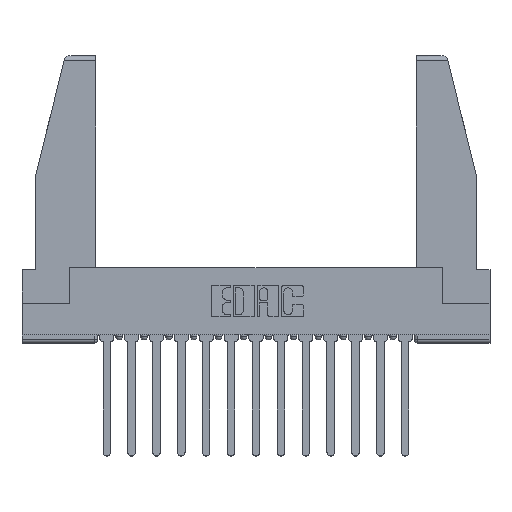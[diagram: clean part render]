
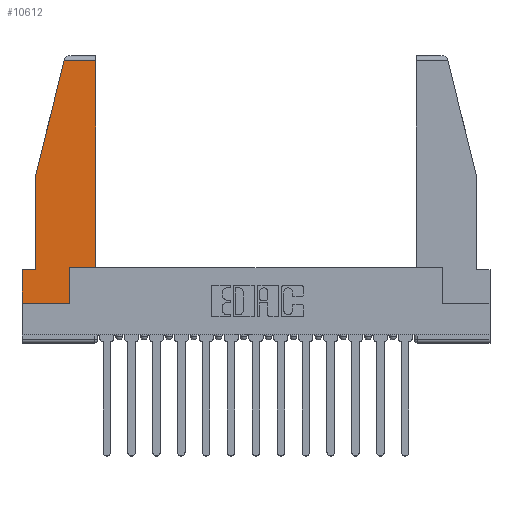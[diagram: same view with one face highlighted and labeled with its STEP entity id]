
A CAD part, top view. The second image highlights one B-rep face of the part: STEP entity #10612.
In plain terms, the highlighted planar face has unit normal (0, 0, 1).
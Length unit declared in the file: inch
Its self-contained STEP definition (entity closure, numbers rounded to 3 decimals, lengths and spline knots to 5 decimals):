
#54 = CARTESIAN_POINT ( 'NONE',  ( 0.086, 0.8, 0. ) ) ;
#259 = VECTOR ( 'NONE', #15701, 39.37008 ) ;
#649 = VECTOR ( 'NONE', #9842, 39.37008 ) ;
#1155 = EDGE_CURVE ( 'NONE', #9492, #9834, #7356, .T. ) ;
#1210 = CARTESIAN_POINT ( 'NONE',  ( 0., 0.21, 0. ) ) ;
#1335 = CARTESIAN_POINT ( 'NONE',  ( 0.086, 0.8, 0. ) ) ;
#1505 = ORIENTED_EDGE ( 'NONE', *, *, #7313, .T. ) ;
#1753 = DIRECTION ( 'NONE',  ( 0., 0., 1. ) ) ;
#2202 = CARTESIAN_POINT ( 'NONE',  ( 0., 0., 0. ) ) ;
#2274 = ORIENTED_EDGE ( 'NONE', *, *, #9126, .T. ) ;
#2557 = CARTESIAN_POINT ( 'NONE',  ( 0.297, 0., 0. ) ) ;
#2591 = VERTEX_POINT ( 'NONE', #7736 ) ;
#2814 = VERTEX_POINT ( 'NONE', #14049 ) ;
#3544 = VECTOR ( 'NONE', #5554, 39.37008 ) ;
#4175 = CARTESIAN_POINT ( 'NONE',  ( 0., 0.21, 0. ) ) ;
#4915 = LINE ( 'NONE', #11040, #16623 ) ;
#5093 = LINE ( 'NONE', #54, #8289 ) ;
#5324 = ORIENTED_EDGE ( 'NONE', *, *, #15727, .T. ) ;
#5519 = CARTESIAN_POINT ( 'NONE',  ( 0.461, 0.223, 0. ) ) ;
#5554 = DIRECTION ( 'NONE',  ( 0., -1., 0. ) ) ;
#5571 = CARTESIAN_POINT ( 'NONE',  ( 0., 1.52, 0. ) ) ;
#5779 = DIRECTION ( 'NONE',  ( 1., 0., 0. ) ) ;
#6099 = FACE_OUTER_BOUND ( 'NONE', #8479, .T. ) ;
#6162 = CARTESIAN_POINT ( 'NONE',  ( 0.086, 0.21, 0. ) ) ;
#6702 = DIRECTION ( 'NONE',  ( -1., 0., 0. ) ) ;
#7313 = EDGE_CURVE ( 'NONE', #2814, #13799, #17312, .T. ) ;
#7356 = LINE ( 'NONE', #4175, #3544 ) ;
#7708 = VERTEX_POINT ( 'NONE', #10818 ) ;
#7736 = CARTESIAN_POINT ( 'NONE',  ( 0.297, 0., 0. ) ) ;
#7889 = ORIENTED_EDGE ( 'NONE', *, *, #16744, .T. ) ;
#7936 = DIRECTION ( 'NONE',  ( 0., 1., 0. ) ) ;
#8087 = VECTOR ( 'NONE', #6702, 39.37008 ) ;
#8289 = VECTOR ( 'NONE', #10872, 39.37008 ) ;
#8439 = CARTESIAN_POINT ( 'NONE',  ( 0., 0.21, 0. ) ) ;
#8461 = LINE ( 'NONE', #15253, #649 ) ;
#8479 = EDGE_LOOP ( 'NONE', ( #2274, #5324, #10916, #12955, #14095, #17023, #15473, #7889, #1505 ) ) ;
#8797 = VECTOR ( 'NONE', #14078, 39.37008 ) ;
#9126 = EDGE_CURVE ( 'NONE', #13799, #16346, #9981, .T. ) ;
#9385 = EDGE_CURVE ( 'NONE', #14887, #15211, #5093, .T. ) ;
#9492 = VERTEX_POINT ( 'NONE', #8439 ) ;
#9834 = VERTEX_POINT ( 'NONE', #2202 ) ;
#9842 = DIRECTION ( 'NONE',  ( -0.239, -0.971, 0. ) ) ;
#9981 = LINE ( 'NONE', #11526, #259 ) ;
#10175 = EDGE_CURVE ( 'NONE', #7708, #14887, #8461, .T. ) ;
#10305 = LINE ( 'NONE', #2557, #11815 ) ;
#10612 = ADVANCED_FACE ( 'NONE', ( #6099 ), #16486, .T. ) ;
#10818 = CARTESIAN_POINT ( 'NONE',  ( 0.2636, 1.52, 0. ) ) ;
#10872 = DIRECTION ( 'NONE',  ( 0., -1., 0. ) ) ;
#10916 = ORIENTED_EDGE ( 'NONE', *, *, #10175, .T. ) ;
#11040 = CARTESIAN_POINT ( 'NONE',  ( 0., 0., 0. ) ) ;
#11102 = DIRECTION ( 'NONE',  ( 1., 0., 0. ) ) ;
#11526 = CARTESIAN_POINT ( 'NONE',  ( 0.461, 0.223, 0. ) ) ;
#11815 = VECTOR ( 'NONE', #7936, 39.37008 ) ;
#12280 = LINE ( 'NONE', #5571, #16309 ) ;
#12955 = ORIENTED_EDGE ( 'NONE', *, *, #9385, .T. ) ;
#13193 = EDGE_CURVE ( 'NONE', #9834, #2591, #4915, .T. ) ;
#13586 = EDGE_CURVE ( 'NONE', #15211, #9492, #13845, .T. ) ;
#13799 = VERTEX_POINT ( 'NONE', #5519 ) ;
#13845 = LINE ( 'NONE', #1210, #8087 ) ;
#14049 = CARTESIAN_POINT ( 'NONE',  ( 0.297, 0.223, 0. ) ) ;
#14078 = DIRECTION ( 'NONE',  ( 1., 0., 0. ) ) ;
#14095 = ORIENTED_EDGE ( 'NONE', *, *, #13586, .T. ) ;
#14887 = VERTEX_POINT ( 'NONE', #1335 ) ;
#15075 = DIRECTION ( 'NONE',  ( -1., 0., 0. ) ) ;
#15114 = AXIS2_PLACEMENT_3D ( 'NONE', #15168, #1753, #5779 ) ;
#15168 = CARTESIAN_POINT ( 'NONE',  ( 0., 0., 0. ) ) ;
#15211 = VERTEX_POINT ( 'NONE', #6162 ) ;
#15253 = CARTESIAN_POINT ( 'NONE',  ( 0.271, 1.55, 0. ) ) ;
#15473 = ORIENTED_EDGE ( 'NONE', *, *, #13193, .T. ) ;
#15668 = CARTESIAN_POINT ( 'NONE',  ( 0.297, 0.223, 0. ) ) ;
#15701 = DIRECTION ( 'NONE',  ( 0., 1., 0. ) ) ;
#15727 = EDGE_CURVE ( 'NONE', #16346, #7708, #12280, .T. ) ;
#16309 = VECTOR ( 'NONE', #15075, 39.37008 ) ;
#16346 = VERTEX_POINT ( 'NONE', #16659 ) ;
#16486 = PLANE ( 'NONE',  #15114 ) ;
#16623 = VECTOR ( 'NONE', #11102, 39.37008 ) ;
#16659 = CARTESIAN_POINT ( 'NONE',  ( 0.461, 1.52, 0. ) ) ;
#16744 = EDGE_CURVE ( 'NONE', #2591, #2814, #10305, .T. ) ;
#17023 = ORIENTED_EDGE ( 'NONE', *, *, #1155, .T. ) ;
#17312 = LINE ( 'NONE', #15668, #8797 ) ;
